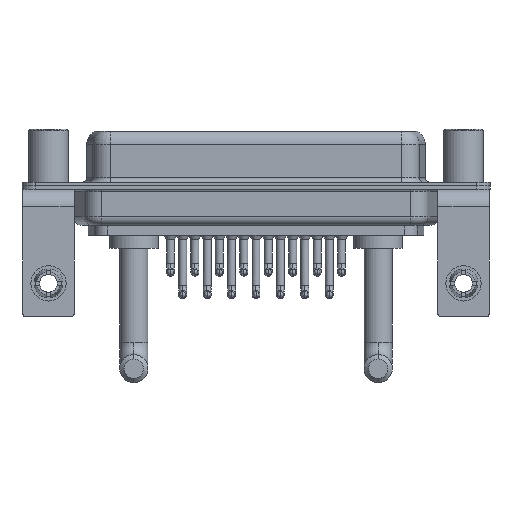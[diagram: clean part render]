
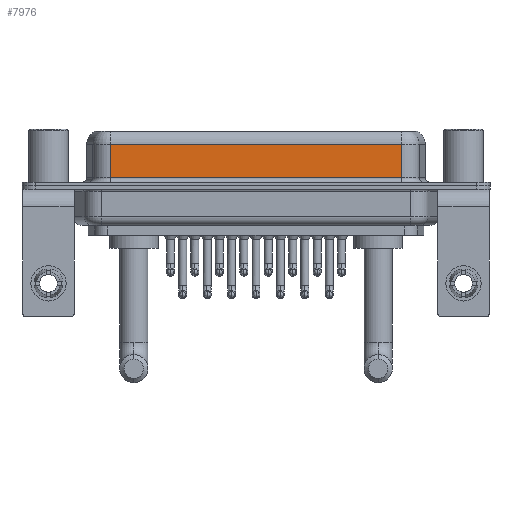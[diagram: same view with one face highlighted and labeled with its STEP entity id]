
A CAD part, front view. The second image highlights one B-rep face of the part: STEP entity #7976.
In plain terms, the highlighted planar face has unit normal (0, -1, 0).
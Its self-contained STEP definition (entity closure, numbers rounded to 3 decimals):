
#711 = CARTESIAN_POINT ( 'NONE',  ( 40.037, -3.95, 4.65 ) ) ;
#739 = CARTESIAN_POINT ( 'NONE',  ( 40.037, -3.95, 6.4 ) ) ;
#871 = VECTOR ( 'NONE', #21977, 1000. ) ;
#1753 = CARTESIAN_POINT ( 'NONE',  ( 40.037, -3.95, 0.9 ) ) ;
#2368 = LINE ( 'NONE', #4504, #12186 ) ;
#3608 = PLANE ( 'NONE',  #7582 ) ;
#4504 = CARTESIAN_POINT ( 'NONE',  ( 7.013, -3.95, 6.4 ) ) ;
#5564 = DIRECTION ( 'NONE',  ( -1., 0., 0. ) ) ;
#6148 = CARTESIAN_POINT ( 'NONE',  ( 7.013, -3.95, 0.9 ) ) ;
#6401 = DIRECTION ( 'NONE',  ( 0., 0., -1. ) ) ;
#6502 = CARTESIAN_POINT ( 'NONE',  ( 40.037, -3.95, 6.4 ) ) ;
#7582 = AXIS2_PLACEMENT_3D ( 'NONE', #6502, #10296, #19666 ) ;
#7887 = VERTEX_POINT ( 'NONE', #19285 ) ;
#7976 = ADVANCED_FACE ( 'NONE', ( #22709 ), #3608, .F. ) ;
#9213 = EDGE_CURVE ( 'NONE', #17239, #7887, #19481, .T. ) ;
#9564 = LINE ( 'NONE', #21328, #24677 ) ;
#10296 = DIRECTION ( 'NONE',  ( 0., 1., 0. ) ) ;
#10708 = ORIENTED_EDGE ( 'NONE', *, *, #9213, .T. ) ;
#12186 = VECTOR ( 'NONE', #6401, 1000. ) ;
#12249 = LINE ( 'NONE', #739, #871 ) ;
#12740 = EDGE_CURVE ( 'NONE', #15058, #20216, #9564, .T. ) ;
#15058 = VERTEX_POINT ( 'NONE', #6148 ) ;
#15428 = EDGE_LOOP ( 'NONE', ( #17230, #10708, #19446, #24162 ) ) ;
#16807 = EDGE_CURVE ( 'NONE', #17239, #20216, #12249, .T. ) ;
#17189 = CARTESIAN_POINT ( 'NONE',  ( 40.037, -3.95, 4.65 ) ) ;
#17230 = ORIENTED_EDGE ( 'NONE', *, *, #16807, .F. ) ;
#17239 = VERTEX_POINT ( 'NONE', #711 ) ;
#17309 = EDGE_CURVE ( 'NONE', #7887, #15058, #2368, .T. ) ;
#19285 = CARTESIAN_POINT ( 'NONE',  ( 7.013, -3.95, 4.65 ) ) ;
#19426 = DIRECTION ( 'NONE',  ( 1., 0., 0. ) ) ;
#19446 = ORIENTED_EDGE ( 'NONE', *, *, #17309, .T. ) ;
#19481 = LINE ( 'NONE', #17189, #21383 ) ;
#19666 = DIRECTION ( 'NONE',  ( 0., 0., 1. ) ) ;
#20216 = VERTEX_POINT ( 'NONE', #1753 ) ;
#21328 = CARTESIAN_POINT ( 'NONE',  ( 40.037, -3.95, 0.9 ) ) ;
#21383 = VECTOR ( 'NONE', #5564, 1000. ) ;
#21977 = DIRECTION ( 'NONE',  ( 0., 0., -1. ) ) ;
#22709 = FACE_OUTER_BOUND ( 'NONE', #15428, .T. ) ;
#24162 = ORIENTED_EDGE ( 'NONE', *, *, #12740, .T. ) ;
#24677 = VECTOR ( 'NONE', #19426, 1000. ) ;
